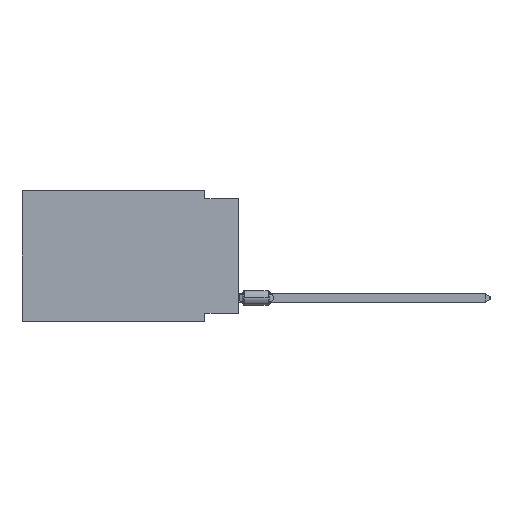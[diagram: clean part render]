
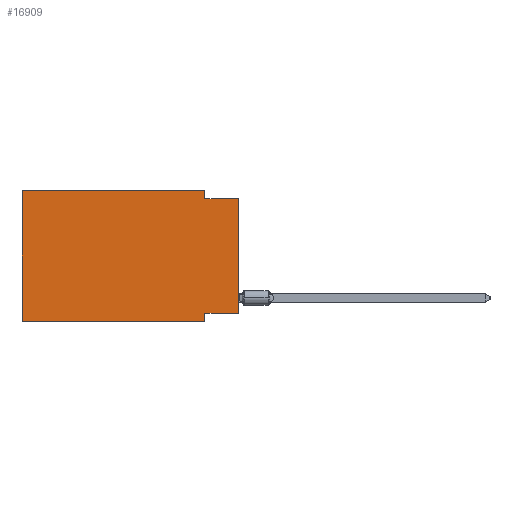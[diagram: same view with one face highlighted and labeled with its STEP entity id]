
A CAD part, left-side view. The second image highlights one B-rep face of the part: STEP entity #16909.
In plain terms, the highlighted planar face has unit normal (-1, 0, 0).
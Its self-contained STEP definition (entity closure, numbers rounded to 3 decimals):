
#5947 = VECTOR ( 'NONE', #31417, 1000. ) ;
#6044 = CARTESIAN_POINT ( 'NONE',  ( 0., 0., -9.271 ) ) ;
#7356 = LINE ( 'NONE', #30312, #5947 ) ;
#11477 = DIRECTION ( 'NONE',  ( 0., 0., -1. ) ) ;
#11745 = DIRECTION ( 'NONE',  ( 0., 0., -1. ) ) ;
#12839 = LINE ( 'NONE', #24119, #72709 ) ;
#13032 = VECTOR ( 'NONE', #11745, 1000. ) ;
#13590 = EDGE_CURVE ( 'NONE', #55189, #48583, #63299, .T. ) ;
#13925 = VERTEX_POINT ( 'NONE', #33480 ) ;
#15990 = DIRECTION ( 'NONE',  ( 1., 0., 0. ) ) ;
#16909 = ADVANCED_FACE ( 'NONE', ( #61914 ), #57365, .F. ) ;
#16948 = LINE ( 'NONE', #23369, #50349 ) ;
#17844 = CARTESIAN_POINT ( 'NONE',  ( 0., 0., -0.635 ) ) ;
#17893 = DIRECTION ( 'NONE',  ( 0., -1., 0. ) ) ;
#18133 = CARTESIAN_POINT ( 'NONE',  ( 0., 2.54, -9.906 ) ) ;
#18480 = LINE ( 'NONE', #6044, #56974 ) ;
#20317 = CARTESIAN_POINT ( 'NONE',  ( 0., 2.54, -0.635 ) ) ;
#20924 = CARTESIAN_POINT ( 'NONE',  ( 0., 0., -9.271 ) ) ;
#22865 = VERTEX_POINT ( 'NONE', #17844 ) ;
#22903 = EDGE_CURVE ( 'NONE', #69377, #22865, #35153, .T. ) ;
#23369 = CARTESIAN_POINT ( 'NONE',  ( 0., 16.383, 0. ) ) ;
#24119 = CARTESIAN_POINT ( 'NONE',  ( 0., 16.383, -9.906 ) ) ;
#24463 = ORIENTED_EDGE ( 'NONE', *, *, #56713, .F. ) ;
#26882 = LINE ( 'NONE', #49858, #64890 ) ;
#27625 = ORIENTED_EDGE ( 'NONE', *, *, #56548, .F. ) ;
#28179 = ORIENTED_EDGE ( 'NONE', *, *, #22903, .T. ) ;
#29760 = DIRECTION ( 'NONE',  ( 0., 1., 0. ) ) ;
#30043 = EDGE_CURVE ( 'NONE', #13925, #48583, #12839, .T. ) ;
#30312 = CARTESIAN_POINT ( 'NONE',  ( 0., 16.383, 0. ) ) ;
#31417 = DIRECTION ( 'NONE',  ( 0., 0., 1. ) ) ;
#31873 = VERTEX_POINT ( 'NONE', #44322 ) ;
#33480 = CARTESIAN_POINT ( 'NONE',  ( 0., 16.383, -9.906 ) ) ;
#35153 = LINE ( 'NONE', #38027, #35576 ) ;
#35407 = DIRECTION ( 'NONE',  ( 0., -1., 0. ) ) ;
#35576 = VECTOR ( 'NONE', #38379, 1000. ) ;
#37525 = ORIENTED_EDGE ( 'NONE', *, *, #55182, .F. ) ;
#38027 = CARTESIAN_POINT ( 'NONE',  ( 0., 0., 0. ) ) ;
#38379 = DIRECTION ( 'NONE',  ( 0., 0., 1. ) ) ;
#44322 = CARTESIAN_POINT ( 'NONE',  ( 0., 16.383, 0. ) ) ;
#45241 = EDGE_CURVE ( 'NONE', #69377, #55189, #18480, .T. ) ;
#48583 = VERTEX_POINT ( 'NONE', #65966 ) ;
#49858 = CARTESIAN_POINT ( 'NONE',  ( 0., 2.54, 0. ) ) ;
#49892 = VERTEX_POINT ( 'NONE', #68567 ) ;
#50349 = VECTOR ( 'NONE', #35407, 1000. ) ;
#51963 = CARTESIAN_POINT ( 'NONE',  ( 0., 2.54, -9.271 ) ) ;
#52559 = ORIENTED_EDGE ( 'NONE', *, *, #30043, .T. ) ;
#55182 = EDGE_CURVE ( 'NONE', #31873, #49892, #16948, .T. ) ;
#55189 = VERTEX_POINT ( 'NONE', #51963 ) ;
#56548 = EDGE_CURVE ( 'NONE', #58835, #22865, #68687, .T. ) ;
#56565 = ORIENTED_EDGE ( 'NONE', *, *, #57842, .F. ) ;
#56713 = EDGE_CURVE ( 'NONE', #49892, #58835, #26882, .T. ) ;
#56974 = VECTOR ( 'NONE', #29760, 1000. ) ;
#57365 = PLANE ( 'NONE',  #63836 ) ;
#57842 = EDGE_CURVE ( 'NONE', #13925, #31873, #7356, .T. ) ;
#58280 = EDGE_LOOP ( 'NONE', ( #28179, #27625, #24463, #37525, #56565, #52559, #70835, #72764 ) ) ;
#58835 = VERTEX_POINT ( 'NONE', #20317 ) ;
#61235 = VECTOR ( 'NONE', #17893, 1000. ) ;
#61914 = FACE_OUTER_BOUND ( 'NONE', #58280, .T. ) ;
#63299 = LINE ( 'NONE', #18133, #13032 ) ;
#63836 = AXIS2_PLACEMENT_3D ( 'NONE', #73553, #15990, #11477 ) ;
#64890 = VECTOR ( 'NONE', #72789, 1000. ) ;
#65966 = CARTESIAN_POINT ( 'NONE',  ( 0., 2.54, -9.906 ) ) ;
#68567 = CARTESIAN_POINT ( 'NONE',  ( 0., 2.54, 0. ) ) ;
#68687 = LINE ( 'NONE', #69442, #61235 ) ;
#69377 = VERTEX_POINT ( 'NONE', #20924 ) ;
#69442 = CARTESIAN_POINT ( 'NONE',  ( 0., 0., -0.635 ) ) ;
#70398 = DIRECTION ( 'NONE',  ( 0., -1., 0. ) ) ;
#70835 = ORIENTED_EDGE ( 'NONE', *, *, #13590, .F. ) ;
#72709 = VECTOR ( 'NONE', #70398, 1000. ) ;
#72764 = ORIENTED_EDGE ( 'NONE', *, *, #45241, .F. ) ;
#72789 = DIRECTION ( 'NONE',  ( 0., 0., -1. ) ) ;
#73553 = CARTESIAN_POINT ( 'NONE',  ( 0., 16.383, 0. ) ) ;
